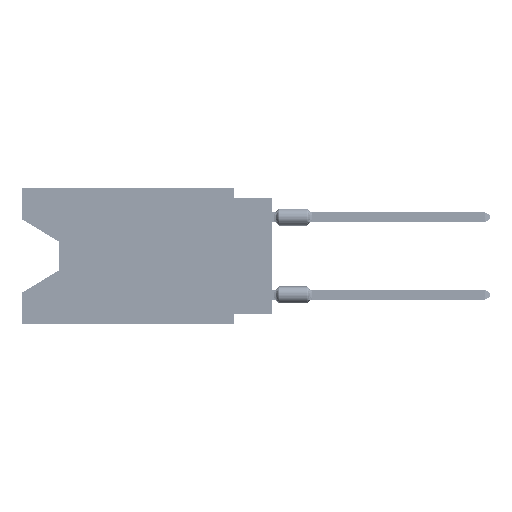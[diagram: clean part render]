
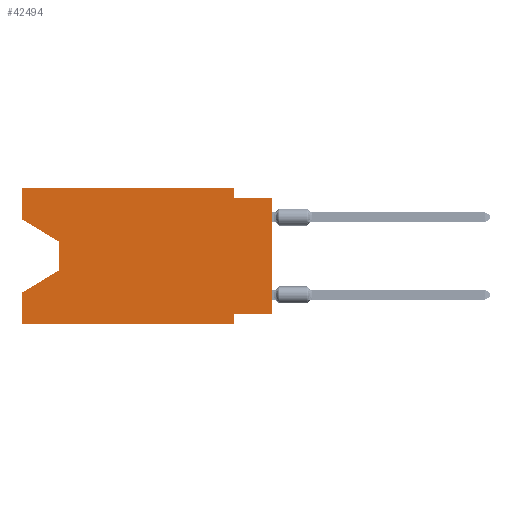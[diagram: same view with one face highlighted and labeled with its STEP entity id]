
A CAD part, left-side view. The second image highlights one B-rep face of the part: STEP entity #42494.
In plain terms, the highlighted planar face has unit normal (-1, 0, 0).
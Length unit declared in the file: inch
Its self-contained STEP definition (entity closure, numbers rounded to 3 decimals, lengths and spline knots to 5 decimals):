
#531 = VECTOR ( 'NONE', #57552, 39.37008 ) ;
#1747 = CARTESIAN_POINT ( 'NONE',  ( 0., 0.1, 0. ) ) ;
#1822 = CARTESIAN_POINT ( 'NONE',  ( 0., 0.55, -0.212 ) ) ;
#2298 = EDGE_CURVE ( 'NONE', #67929, #96060, #13025, .T. ) ;
#2761 = CARTESIAN_POINT ( 'NONE',  ( 0., 0.645, -0.26975 ) ) ;
#3573 = EDGE_CURVE ( 'NONE', #9168, #21777, #30443, .T. ) ;
#3836 = ORIENTED_EDGE ( 'NONE', *, *, #63277, .T. ) ;
#5678 = VERTEX_POINT ( 'NONE', #83263 ) ;
#8194 = ORIENTED_EDGE ( 'NONE', *, *, #64045, .F. ) ;
#8326 = DIRECTION ( 'NONE',  ( 0., 0.855, -0.519 ) ) ;
#9168 = VERTEX_POINT ( 'NONE', #53933 ) ;
#9687 = FACE_OUTER_BOUND ( 'NONE', #49977, .T. ) ;
#10811 = CARTESIAN_POINT ( 'NONE',  ( 0., 0.645, 0. ) ) ;
#12071 = VERTEX_POINT ( 'NONE', #1822 ) ;
#12450 = CARTESIAN_POINT ( 'NONE',  ( 0., 0., -0.025 ) ) ;
#13025 = LINE ( 'NONE', #12450, #33166 ) ;
#13208 = ORIENTED_EDGE ( 'NONE', *, *, #2298, .F. ) ;
#14104 = LINE ( 'NONE', #57408, #109142 ) ;
#16765 = VERTEX_POINT ( 'NONE', #102451 ) ;
#16976 = CARTESIAN_POINT ( 'NONE',  ( 0., 0.55, -0.138 ) ) ;
#21777 = VERTEX_POINT ( 'NONE', #95916 ) ;
#25357 = CARTESIAN_POINT ( 'NONE',  ( 0., 0.645, 0. ) ) ;
#25595 = CARTESIAN_POINT ( 'NONE',  ( 0., 0.1, -0.35 ) ) ;
#29591 = LINE ( 'NONE', #64766, #90676 ) ;
#30162 = LINE ( 'NONE', #109206, #75944 ) ;
#30443 = LINE ( 'NONE', #65625, #531 ) ;
#31715 = DIRECTION ( 'NONE',  ( 0., -1., 0. ) ) ;
#31944 = EDGE_CURVE ( 'NONE', #16765, #75489, #44379, .T. ) ;
#33166 = VECTOR ( 'NONE', #92616, 39.37008 ) ;
#36930 = DIRECTION ( 'NONE',  ( 0., 0., -1. ) ) ;
#37015 = EDGE_CURVE ( 'NONE', #49603, #96060, #41446, .T. ) ;
#37047 = VECTOR ( 'NONE', #87094, 39.37008 ) ;
#38449 = ORIENTED_EDGE ( 'NONE', *, *, #68467, .F. ) ;
#39006 = EDGE_CURVE ( 'NONE', #5678, #12071, #78684, .T. ) ;
#39490 = CARTESIAN_POINT ( 'NONE',  ( 0., 0.1, 0. ) ) ;
#40084 = DIRECTION ( 'NONE',  ( 0., -1., 0. ) ) ;
#41305 = VERTEX_POINT ( 'NONE', #66256 ) ;
#41446 = LINE ( 'NONE', #42591, #78616 ) ;
#42494 = ADVANCED_FACE ( 'NONE', ( #9687 ), #71404, .F. ) ;
#42591 = CARTESIAN_POINT ( 'NONE',  ( 0., 0., 0. ) ) ;
#42800 = CARTESIAN_POINT ( 'NONE',  ( 0., 0.1, -0.025 ) ) ;
#43204 = VECTOR ( 'NONE', #8326, 39.37008 ) ;
#44379 = LINE ( 'NONE', #25357, #37047 ) ;
#49603 = VERTEX_POINT ( 'NONE', #84229 ) ;
#49611 = ORIENTED_EDGE ( 'NONE', *, *, #68717, .T. ) ;
#49977 = EDGE_LOOP ( 'NONE', ( #76025, #60692, #49611, #108103, #3836, #38449, #8194, #88585, #13208, #100643, #58064, #81564 ) ) ;
#53933 = CARTESIAN_POINT ( 'NONE',  ( 0., 0.645, -0.08025 ) ) ;
#57408 = CARTESIAN_POINT ( 'NONE',  ( 0., 0.645, 0. ) ) ;
#57552 = DIRECTION ( 'NONE',  ( 0., 0., 1. ) ) ;
#58064 = ORIENTED_EDGE ( 'NONE', *, *, #66106, .F. ) ;
#60692 = ORIENTED_EDGE ( 'NONE', *, *, #39006, .T. ) ;
#62424 = VERTEX_POINT ( 'NONE', #39490 ) ;
#63277 = EDGE_CURVE ( 'NONE', #16765, #81422, #99817, .T. ) ;
#64045 = EDGE_CURVE ( 'NONE', #49603, #41305, #29591, .T. ) ;
#64137 = EDGE_CURVE ( 'NONE', #9168, #5678, #30162, .T. ) ;
#64449 = DIRECTION ( 'NONE',  ( 0., 0., -1. ) ) ;
#64616 = CARTESIAN_POINT ( 'NONE',  ( 0., 0.645, -0.35 ) ) ;
#64766 = CARTESIAN_POINT ( 'NONE',  ( 0., 0., -0.325 ) ) ;
#65625 = CARTESIAN_POINT ( 'NONE',  ( 0., 0.645, 0. ) ) ;
#66106 = EDGE_CURVE ( 'NONE', #21777, #62424, #14104, .T. ) ;
#66256 = CARTESIAN_POINT ( 'NONE',  ( 0., 0.1, -0.325 ) ) ;
#67929 = VERTEX_POINT ( 'NONE', #42800 ) ;
#68467 = EDGE_CURVE ( 'NONE', #41305, #81422, #81131, .T. ) ;
#68717 = EDGE_CURVE ( 'NONE', #12071, #75489, #104702, .T. ) ;
#71404 = PLANE ( 'NONE',  #86585 ) ;
#71996 = CARTESIAN_POINT ( 'NONE',  ( 0., 0., -0.025 ) ) ;
#73469 = VECTOR ( 'NONE', #36930, 39.37008 ) ;
#75489 = VERTEX_POINT ( 'NONE', #2761 ) ;
#75707 = DIRECTION ( 'NONE',  ( 0., -0.855, -0.519 ) ) ;
#75944 = VECTOR ( 'NONE', #75707, 39.37008 ) ;
#76025 = ORIENTED_EDGE ( 'NONE', *, *, #64137, .T. ) ;
#78616 = VECTOR ( 'NONE', #87009, 39.37008 ) ;
#78684 = LINE ( 'NONE', #16976, #91533 ) ;
#79294 = CARTESIAN_POINT ( 'NONE',  ( 0., 0.55, -0.212 ) ) ;
#80025 = VECTOR ( 'NONE', #98446, 39.37008 ) ;
#80546 = CARTESIAN_POINT ( 'NONE',  ( 0., 0.1, -0.35 ) ) ;
#80606 = DIRECTION ( 'NONE',  ( 1., 0., 0. ) ) ;
#80750 = LINE ( 'NONE', #1747, #73469 ) ;
#81131 = LINE ( 'NONE', #80546, #80025 ) ;
#81422 = VERTEX_POINT ( 'NONE', #25595 ) ;
#81564 = ORIENTED_EDGE ( 'NONE', *, *, #3573, .F. ) ;
#83263 = CARTESIAN_POINT ( 'NONE',  ( 0., 0.55, -0.138 ) ) ;
#84229 = CARTESIAN_POINT ( 'NONE',  ( 0., 0., -0.325 ) ) ;
#86585 = AXIS2_PLACEMENT_3D ( 'NONE', #10811, #80606, #64449 ) ;
#87009 = DIRECTION ( 'NONE',  ( 0., 0., 1. ) ) ;
#87094 = DIRECTION ( 'NONE',  ( 0., 0., 1. ) ) ;
#87349 = DIRECTION ( 'NONE',  ( 0., 0., -1. ) ) ;
#88585 = ORIENTED_EDGE ( 'NONE', *, *, #37015, .T. ) ;
#88713 = VECTOR ( 'NONE', #31715, 39.37008 ) ;
#90676 = VECTOR ( 'NONE', #98816, 39.37008 ) ;
#91533 = VECTOR ( 'NONE', #87349, 39.37008 ) ;
#92616 = DIRECTION ( 'NONE',  ( 0., -1., 0. ) ) ;
#95916 = CARTESIAN_POINT ( 'NONE',  ( 0., 0.645, 0. ) ) ;
#96060 = VERTEX_POINT ( 'NONE', #71996 ) ;
#98446 = DIRECTION ( 'NONE',  ( 0., 0., -1. ) ) ;
#98816 = DIRECTION ( 'NONE',  ( 0., 1., 0. ) ) ;
#99817 = LINE ( 'NONE', #64616, #88713 ) ;
#100643 = ORIENTED_EDGE ( 'NONE', *, *, #108977, .F. ) ;
#102451 = CARTESIAN_POINT ( 'NONE',  ( 0., 0.645, -0.35 ) ) ;
#104702 = LINE ( 'NONE', #79294, #43204 ) ;
#108103 = ORIENTED_EDGE ( 'NONE', *, *, #31944, .F. ) ;
#108977 = EDGE_CURVE ( 'NONE', #62424, #67929, #80750, .T. ) ;
#109142 = VECTOR ( 'NONE', #40084, 39.37008 ) ;
#109206 = CARTESIAN_POINT ( 'NONE',  ( 0., 0.645, -0.08025 ) ) ;
